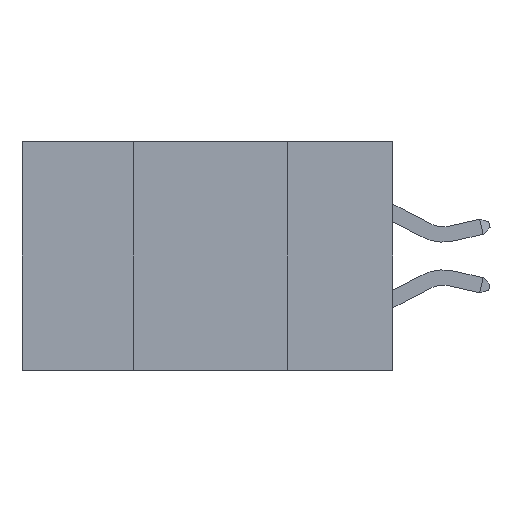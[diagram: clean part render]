
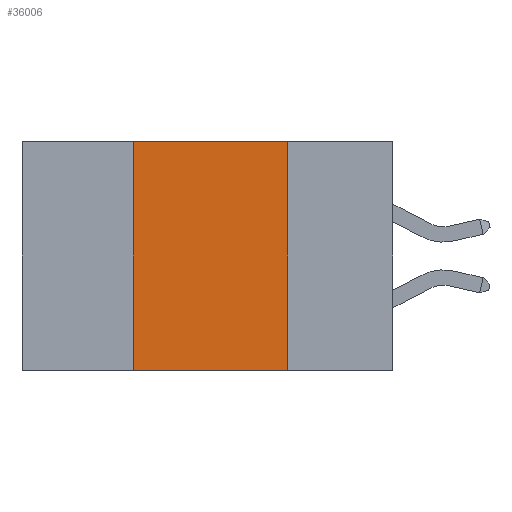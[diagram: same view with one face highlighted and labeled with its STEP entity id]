
A CAD part, left-side view. The second image highlights one B-rep face of the part: STEP entity #36006.
In plain terms, the highlighted planar face has unit normal (-1, 0, 0).
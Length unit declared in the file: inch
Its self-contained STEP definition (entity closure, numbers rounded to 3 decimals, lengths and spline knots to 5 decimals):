
#1217 = DIRECTION ( 'NONE',  ( 0., 0., -1. ) ) ;
#2145 = DIRECTION ( 'NONE',  ( 0., -1., 0. ) ) ;
#2588 = EDGE_CURVE ( 'NONE', #34896, #17021, #4998, .T. ) ;
#4387 = DIRECTION ( 'NONE',  ( 1., 0., 0. ) ) ;
#4532 = LINE ( 'NONE', #13676, #10164 ) ;
#4577 = ORIENTED_EDGE ( 'NONE', *, *, #37163, .F. ) ;
#4998 = LINE ( 'NONE', #16653, #12812 ) ;
#10164 = VECTOR ( 'NONE', #13303, 39.37008 ) ;
#12194 = DIRECTION ( 'NONE',  ( 0., 0., 1. ) ) ;
#12812 = VECTOR ( 'NONE', #2145, 39.37008 ) ;
#13031 = LINE ( 'NONE', #29784, #21545 ) ;
#13303 = DIRECTION ( 'NONE',  ( 0., -1., 0. ) ) ;
#13432 = EDGE_CURVE ( 'NONE', #36974, #27432, #4532, .T. ) ;
#13676 = CARTESIAN_POINT ( 'NONE',  ( 0., 0.6, -0.37 ) ) ;
#16002 = ORIENTED_EDGE ( 'NONE', *, *, #13432, .T. ) ;
#16653 = CARTESIAN_POINT ( 'NONE',  ( 0., 0.6, 0. ) ) ;
#17021 = VERTEX_POINT ( 'NONE', #24865 ) ;
#17926 = LINE ( 'NONE', #26673, #36923 ) ;
#18892 = CARTESIAN_POINT ( 'NONE',  ( 0., 0.6, 0. ) ) ;
#19079 = FACE_OUTER_BOUND ( 'NONE', #37514, .T. ) ;
#21523 = ORIENTED_EDGE ( 'NONE', *, *, #27867, .F. ) ;
#21545 = VECTOR ( 'NONE', #1217, 39.37008 ) ;
#22797 = CARTESIAN_POINT ( 'NONE',  ( 0., 0.42, -0.37 ) ) ;
#24865 = CARTESIAN_POINT ( 'NONE',  ( 0., 0.17, 0. ) ) ;
#26673 = CARTESIAN_POINT ( 'NONE',  ( 0., 0.42, 0. ) ) ;
#27432 = VERTEX_POINT ( 'NONE', #32413 ) ;
#27624 = DIRECTION ( 'NONE',  ( 0., 0., -1. ) ) ;
#27867 = EDGE_CURVE ( 'NONE', #36974, #34896, #17926, .T. ) ;
#29784 = CARTESIAN_POINT ( 'NONE',  ( 0., 0.17, 0. ) ) ;
#30675 = PLANE ( 'NONE',  #34263 ) ;
#32175 = CARTESIAN_POINT ( 'NONE',  ( 0., 0.42, 0. ) ) ;
#32413 = CARTESIAN_POINT ( 'NONE',  ( 0., 0.17, -0.37 ) ) ;
#32917 = ORIENTED_EDGE ( 'NONE', *, *, #2588, .F. ) ;
#34263 = AXIS2_PLACEMENT_3D ( 'NONE', #18892, #4387, #27624 ) ;
#34896 = VERTEX_POINT ( 'NONE', #32175 ) ;
#36006 = ADVANCED_FACE ( 'NONE', ( #19079 ), #30675, .F. ) ;
#36923 = VECTOR ( 'NONE', #12194, 39.37008 ) ;
#36974 = VERTEX_POINT ( 'NONE', #22797 ) ;
#37163 = EDGE_CURVE ( 'NONE', #17021, #27432, #13031, .T. ) ;
#37514 = EDGE_LOOP ( 'NONE', ( #4577, #32917, #21523, #16002 ) ) ;
